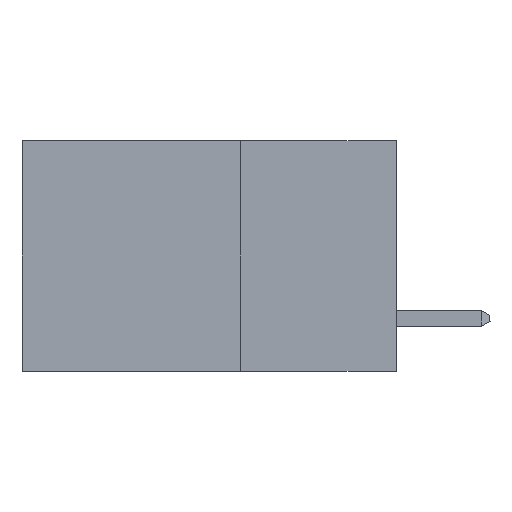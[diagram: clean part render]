
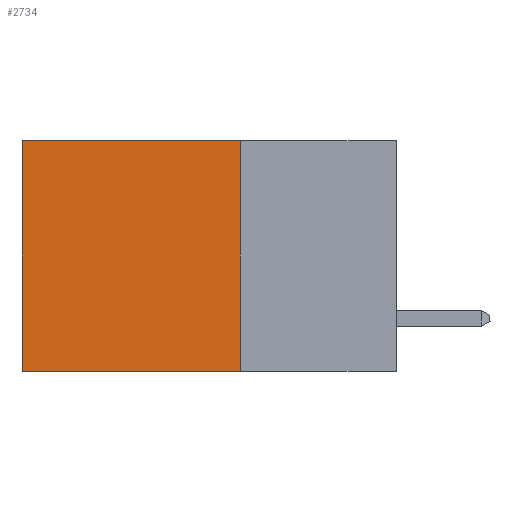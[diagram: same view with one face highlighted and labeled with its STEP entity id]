
A CAD part, left-side view. The second image highlights one B-rep face of the part: STEP entity #2734.
In plain terms, the highlighted planar face has unit normal (-1, 0, 0).
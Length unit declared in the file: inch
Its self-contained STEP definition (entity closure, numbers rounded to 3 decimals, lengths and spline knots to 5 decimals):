
#103 = EDGE_CURVE ( 'NONE', #1767, #8364, #663, .T. ) ;
#389 = CARTESIAN_POINT ( 'NONE',  ( 0.298, 0.6, -0.37 ) ) ;
#663 = LINE ( 'NONE', #2600, #14443 ) ;
#1767 = VERTEX_POINT ( 'NONE', #11321 ) ;
#2046 = VERTEX_POINT ( 'NONE', #389 ) ;
#2472 = CARTESIAN_POINT ( 'NONE',  ( 0.298, 0.6, 0. ) ) ;
#2536 = DIRECTION ( 'NONE',  ( 0., 0., -1. ) ) ;
#2600 = CARTESIAN_POINT ( 'NONE',  ( 0.298, 0.25, 0. ) ) ;
#2651 = LINE ( 'NONE', #15594, #9547 ) ;
#2734 = ADVANCED_FACE ( 'NONE', ( #13104 ), #9114, .F. ) ;
#5639 = AXIS2_PLACEMENT_3D ( 'NONE', #12821, #13692, #12948 ) ;
#6316 = CARTESIAN_POINT ( 'NONE',  ( 0.298, 0.25, -0.37 ) ) ;
#6546 = ORIENTED_EDGE ( 'NONE', *, *, #9482, .T. ) ;
#7014 = EDGE_LOOP ( 'NONE', ( #12974, #10052, #12483, #6546 ) ) ;
#8364 = VERTEX_POINT ( 'NONE', #10197 ) ;
#9082 = VECTOR ( 'NONE', #2536, 39.37008 ) ;
#9114 = PLANE ( 'NONE',  #5639 ) ;
#9243 = LINE ( 'NONE', #6316, #9704 ) ;
#9482 = EDGE_CURVE ( 'NONE', #1767, #11368, #2651, .T. ) ;
#9509 = EDGE_CURVE ( 'NONE', #11368, #2046, #16784, .T. ) ;
#9547 = VECTOR ( 'NONE', #9726, 39.37008 ) ;
#9704 = VECTOR ( 'NONE', #16476, 39.37008 ) ;
#9726 = DIRECTION ( 'NONE',  ( 0., 1., 0. ) ) ;
#10052 = ORIENTED_EDGE ( 'NONE', *, *, #13727, .F. ) ;
#10197 = CARTESIAN_POINT ( 'NONE',  ( 0.298, 0.25, -0.37 ) ) ;
#11321 = CARTESIAN_POINT ( 'NONE',  ( 0.298, 0.25, 0. ) ) ;
#11368 = VERTEX_POINT ( 'NONE', #13874 ) ;
#12483 = ORIENTED_EDGE ( 'NONE', *, *, #103, .F. ) ;
#12821 = CARTESIAN_POINT ( 'NONE',  ( 0.298, 0.25, 0. ) ) ;
#12948 = DIRECTION ( 'NONE',  ( 0., 0., -1. ) ) ;
#12974 = ORIENTED_EDGE ( 'NONE', *, *, #9509, .T. ) ;
#13104 = FACE_OUTER_BOUND ( 'NONE', #7014, .T. ) ;
#13692 = DIRECTION ( 'NONE',  ( 1., 0., 0. ) ) ;
#13727 = EDGE_CURVE ( 'NONE', #8364, #2046, #9243, .T. ) ;
#13874 = CARTESIAN_POINT ( 'NONE',  ( 0.298, 0.6, 0. ) ) ;
#14443 = VECTOR ( 'NONE', #16779, 39.37008 ) ;
#15594 = CARTESIAN_POINT ( 'NONE',  ( 0.298, 0.25, 0. ) ) ;
#16476 = DIRECTION ( 'NONE',  ( 0., 1., 0. ) ) ;
#16779 = DIRECTION ( 'NONE',  ( 0., 0., -1. ) ) ;
#16784 = LINE ( 'NONE', #2472, #9082 ) ;
